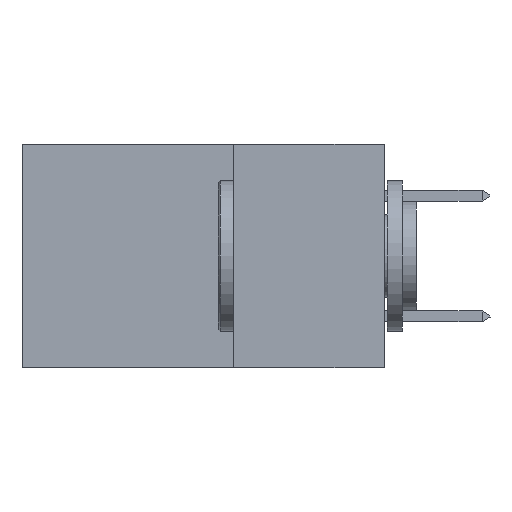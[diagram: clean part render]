
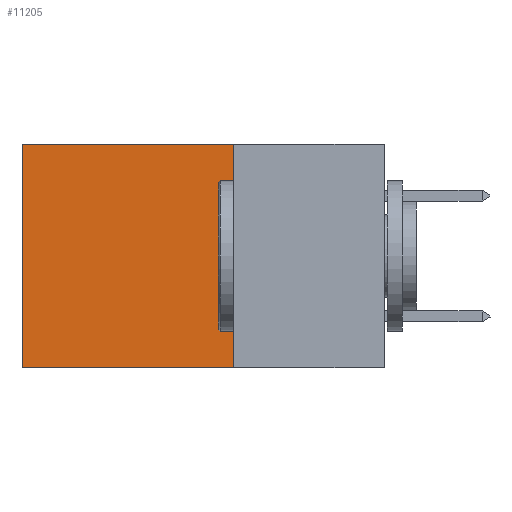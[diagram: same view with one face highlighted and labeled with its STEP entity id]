
A CAD part, left-side view. The second image highlights one B-rep face of the part: STEP entity #11205.
In plain terms, the highlighted planar face has unit normal (-1, 0, 0).
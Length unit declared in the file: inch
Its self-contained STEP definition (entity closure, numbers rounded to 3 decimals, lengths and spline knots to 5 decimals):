
#141 = ORIENTED_EDGE ( 'NONE', *, *, #16097, .T. ) ;
#630 = ORIENTED_EDGE ( 'NONE', *, *, #14962, .T. ) ;
#922 = VECTOR ( 'NONE', #8177, 39.37008 ) ;
#1032 = VERTEX_POINT ( 'NONE', #12490 ) ;
#1252 = CARTESIAN_POINT ( 'NONE',  ( 0.2875, 0.25, 0. ) ) ;
#3313 = VERTEX_POINT ( 'NONE', #14933 ) ;
#3578 = VECTOR ( 'NONE', #7828, 39.37008 ) ;
#3861 = PLANE ( 'NONE',  #10726 ) ;
#4527 = CARTESIAN_POINT ( 'NONE',  ( 0.2875, 0.6, 0. ) ) ;
#5027 = VECTOR ( 'NONE', #5789, 39.37008 ) ;
#5148 = DIRECTION ( 'NONE',  ( 0., 0., -1. ) ) ;
#5231 = CARTESIAN_POINT ( 'NONE',  ( 0.2875, 0.25, -0.37 ) ) ;
#5789 = DIRECTION ( 'NONE',  ( 0., 0., -1. ) ) ;
#6017 = VECTOR ( 'NONE', #7293, 39.37008 ) ;
#6082 = CARTESIAN_POINT ( 'NONE',  ( 0.2875, 0.25, 0. ) ) ;
#6433 = EDGE_CURVE ( 'NONE', #1032, #13647, #7644, .T. ) ;
#7140 = EDGE_CURVE ( 'NONE', #13647, #3313, #12679, .T. ) ;
#7293 = DIRECTION ( 'NONE',  ( 0., 1., 0. ) ) ;
#7365 = CARTESIAN_POINT ( 'NONE',  ( 0.2875, 0.6, 0. ) ) ;
#7383 = ORIENTED_EDGE ( 'NONE', *, *, #7140, .F. ) ;
#7446 = EDGE_LOOP ( 'NONE', ( #141, #7383, #10883, #630 ) ) ;
#7644 = LINE ( 'NONE', #8122, #922 ) ;
#7828 = DIRECTION ( 'NONE',  ( 0., 1., 0. ) ) ;
#8122 = CARTESIAN_POINT ( 'NONE',  ( 0.2875, 0.25, 0. ) ) ;
#8177 = DIRECTION ( 'NONE',  ( 0., 0., -1. ) ) ;
#8191 = CARTESIAN_POINT ( 'NONE',  ( 0.2875, 0.25, -0.37 ) ) ;
#8619 = LINE ( 'NONE', #4527, #5027 ) ;
#10726 = AXIS2_PLACEMENT_3D ( 'NONE', #1252, #12529, #5148 ) ;
#10883 = ORIENTED_EDGE ( 'NONE', *, *, #6433, .F. ) ;
#11119 = VERTEX_POINT ( 'NONE', #7365 ) ;
#11205 = ADVANCED_FACE ( 'NONE', ( #14281 ), #3861, .F. ) ;
#12490 = CARTESIAN_POINT ( 'NONE',  ( 0.2875, 0.25, 0. ) ) ;
#12529 = DIRECTION ( 'NONE',  ( 1., 0., 0. ) ) ;
#12575 = LINE ( 'NONE', #6082, #6017 ) ;
#12679 = LINE ( 'NONE', #8191, #3578 ) ;
#13647 = VERTEX_POINT ( 'NONE', #5231 ) ;
#14281 = FACE_OUTER_BOUND ( 'NONE', #7446, .T. ) ;
#14933 = CARTESIAN_POINT ( 'NONE',  ( 0.2875, 0.6, -0.37 ) ) ;
#14962 = EDGE_CURVE ( 'NONE', #1032, #11119, #12575, .T. ) ;
#16097 = EDGE_CURVE ( 'NONE', #11119, #3313, #8619, .T. ) ;
